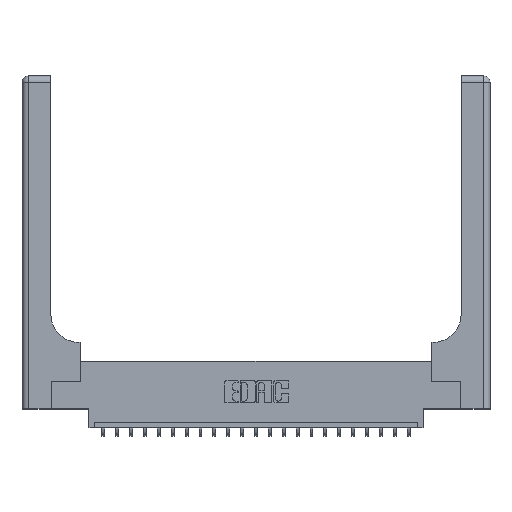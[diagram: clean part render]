
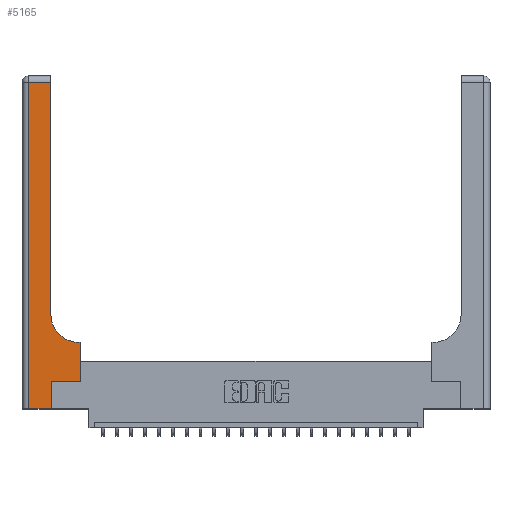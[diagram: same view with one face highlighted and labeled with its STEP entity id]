
A CAD part, top view. The second image highlights one B-rep face of the part: STEP entity #5165.
In plain terms, the highlighted planar face has unit normal (0, 0, 1).
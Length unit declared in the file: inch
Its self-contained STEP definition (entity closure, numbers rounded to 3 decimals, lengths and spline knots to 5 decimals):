
#20 = EDGE_CURVE ( 'NONE', #14560, #20317, #5121, .T. ) ;
#424 = CARTESIAN_POINT ( 'NONE',  ( 0.265, 0., 0.37 ) ) ;
#556 = VECTOR ( 'NONE', #9719, 39.37008 ) ;
#959 = DIRECTION ( 'NONE',  ( -1., 0., 0. ) ) ;
#1201 = LINE ( 'NONE', #4534, #18934 ) ;
#2152 = DIRECTION ( 'NONE',  ( 0., 1., 0. ) ) ;
#2357 = VERTEX_POINT ( 'NONE', #4241 ) ;
#2585 = VECTOR ( 'NONE', #22104, 39.37008 ) ;
#2596 = PLANE ( 'NONE',  #11357 ) ;
#2863 = VERTEX_POINT ( 'NONE', #9606 ) ;
#2919 = CARTESIAN_POINT ( 'NONE',  ( 0.51, 0.85, 0.37 ) ) ;
#2948 = ORIENTED_EDGE ( 'NONE', *, *, #5925, .T. ) ;
#3446 = VERTEX_POINT ( 'NONE', #12946 ) ;
#4241 = CARTESIAN_POINT ( 'NONE',  ( 0.26, 0.85, 0.37 ) ) ;
#4312 = ORIENTED_EDGE ( 'NONE', *, *, #17165, .T. ) ;
#4534 = CARTESIAN_POINT ( 'NONE',  ( 0., 0., 0.37 ) ) ;
#4657 = DIRECTION ( 'NONE',  ( 1., 0., 0. ) ) ;
#5121 = LINE ( 'NONE', #11431, #556 ) ;
#5165 = ADVANCED_FACE ( 'NONE', ( #8249 ), #2596, .F. ) ;
#5503 = EDGE_CURVE ( 'NONE', #7961, #2863, #1201, .T. ) ;
#5925 = EDGE_CURVE ( 'NONE', #13502, #14560, #19758, .T. ) ;
#6110 = CARTESIAN_POINT ( 'NONE',  ( 0.06, 3., 0.37 ) ) ;
#6537 = CARTESIAN_POINT ( 'NONE',  ( 0.26, 2.94, 0.37 ) ) ;
#7366 = LINE ( 'NONE', #21053, #11388 ) ;
#7414 = DIRECTION ( 'NONE',  ( 1., 0., 0. ) ) ;
#7770 = LINE ( 'NONE', #424, #20345 ) ;
#7831 = CARTESIAN_POINT ( 'NONE',  ( 0., 3., 0.37 ) ) ;
#7961 = VERTEX_POINT ( 'NONE', #21617 ) ;
#8249 = FACE_OUTER_BOUND ( 'NONE', #15138, .T. ) ;
#8421 = CARTESIAN_POINT ( 'NONE',  ( 0.26, 3., 0.37 ) ) ;
#9110 = DIRECTION ( 'NONE',  ( -1., 0., 0. ) ) ;
#9540 = DIRECTION ( 'NONE',  ( 0., -1., 0. ) ) ;
#9606 = CARTESIAN_POINT ( 'NONE',  ( 0.265, 0., 0.37 ) ) ;
#9709 = CARTESIAN_POINT ( 'NONE',  ( 0.06, 2.94, 0.37 ) ) ;
#9719 = DIRECTION ( 'NONE',  ( -1., 0., 0. ) ) ;
#10455 = ORIENTED_EDGE ( 'NONE', *, *, #17880, .T. ) ;
#11282 = DIRECTION ( 'NONE',  ( 0., 0., -1. ) ) ;
#11357 = AXIS2_PLACEMENT_3D ( 'NONE', #7831, #11282, #959 ) ;
#11388 = VECTOR ( 'NONE', #9110, 39.37008 ) ;
#11431 = CARTESIAN_POINT ( 'NONE',  ( 0.26, 0.6, 0.37 ) ) ;
#11460 = CARTESIAN_POINT ( 'NONE',  ( 0.528, 0.25, 0.37 ) ) ;
#11741 = CARTESIAN_POINT ( 'NONE',  ( 0.51, 0.6, 0.37 ) ) ;
#12100 = ORIENTED_EDGE ( 'NONE', *, *, #16900, .T. ) ;
#12293 = VECTOR ( 'NONE', #9540, 39.37008 ) ;
#12350 = VECTOR ( 'NONE', #7414, 39.37008 ) ;
#12370 = VERTEX_POINT ( 'NONE', #6537 ) ;
#12835 = LINE ( 'NONE', #6110, #12293 ) ;
#12946 = CARTESIAN_POINT ( 'NONE',  ( 0.265, 0.25, 0.37 ) ) ;
#13502 = VERTEX_POINT ( 'NONE', #11460 ) ;
#14301 = CARTESIAN_POINT ( 'NONE',  ( 0.528, 0.25, 0.37 ) ) ;
#14504 = AXIS2_PLACEMENT_3D ( 'NONE', #2919, #14977, #4657 ) ;
#14560 = VERTEX_POINT ( 'NONE', #17567 ) ;
#14977 = DIRECTION ( 'NONE',  ( 0., 0., -1. ) ) ;
#15138 = EDGE_LOOP ( 'NONE', ( #10455, #20078, #18770, #20375, #19043, #12100, #2948, #17500, #4312 ) ) ;
#15233 = VECTOR ( 'NONE', #21079, 39.37008 ) ;
#15901 = CARTESIAN_POINT ( 'NONE',  ( 0.265, 0.25, 0.37 ) ) ;
#16900 = EDGE_CURVE ( 'NONE', #3446, #13502, #21423, .T. ) ;
#17165 = EDGE_CURVE ( 'NONE', #20317, #2357, #21146, .T. ) ;
#17464 = EDGE_CURVE ( 'NONE', #2863, #3446, #7770, .T. ) ;
#17500 = ORIENTED_EDGE ( 'NONE', *, *, #20, .T. ) ;
#17567 = CARTESIAN_POINT ( 'NONE',  ( 0.528, 0.6, 0.37 ) ) ;
#17705 = VERTEX_POINT ( 'NONE', #9709 ) ;
#17880 = EDGE_CURVE ( 'NONE', #2357, #12370, #20850, .T. ) ;
#18297 = EDGE_CURVE ( 'NONE', #17705, #7961, #12835, .T. ) ;
#18770 = ORIENTED_EDGE ( 'NONE', *, *, #18297, .T. ) ;
#18934 = VECTOR ( 'NONE', #21621, 39.37008 ) ;
#19043 = ORIENTED_EDGE ( 'NONE', *, *, #17464, .T. ) ;
#19758 = LINE ( 'NONE', #14301, #15233 ) ;
#20078 = ORIENTED_EDGE ( 'NONE', *, *, #20581, .T. ) ;
#20317 = VERTEX_POINT ( 'NONE', #11741 ) ;
#20345 = VECTOR ( 'NONE', #2152, 39.37008 ) ;
#20375 = ORIENTED_EDGE ( 'NONE', *, *, #5503, .T. ) ;
#20581 = EDGE_CURVE ( 'NONE', #12370, #17705, #7366, .T. ) ;
#20850 = LINE ( 'NONE', #8421, #2585 ) ;
#21053 = CARTESIAN_POINT ( 'NONE',  ( 0., 2.94, 0.37 ) ) ;
#21079 = DIRECTION ( 'NONE',  ( 0., 1., 0. ) ) ;
#21146 = CIRCLE ( 'NONE', #14504, 0.25 ) ;
#21423 = LINE ( 'NONE', #15901, #12350 ) ;
#21617 = CARTESIAN_POINT ( 'NONE',  ( 0.06, 0., 0.37 ) ) ;
#21621 = DIRECTION ( 'NONE',  ( 1., 0., 0. ) ) ;
#22104 = DIRECTION ( 'NONE',  ( 0., 1., 0. ) ) ;
